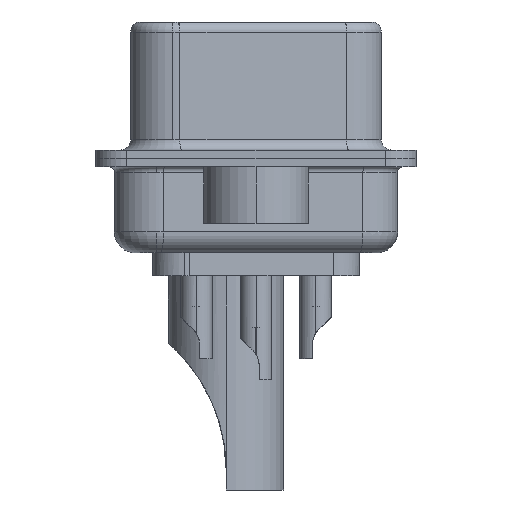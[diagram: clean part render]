
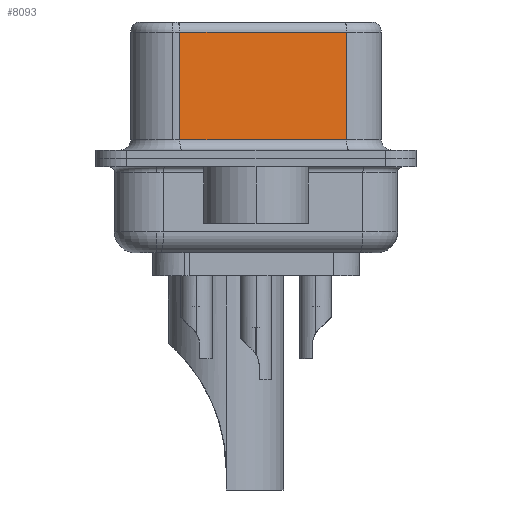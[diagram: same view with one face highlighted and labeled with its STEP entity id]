
A CAD part, left-side view. The second image highlights one B-rep face of the part: STEP entity #8093.
In plain terms, the highlighted planar face has unit normal (-0.985, -0.174, 0).
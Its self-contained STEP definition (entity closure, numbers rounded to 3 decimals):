
#473 = ORIENTED_EDGE ( 'NONE', *, *, #5941, .F. ) ;
#617 = LINE ( 'NONE', #20745, #11961 ) ;
#3370 = DIRECTION ( 'NONE',  ( -0.174, 0.985, 0. ) ) ;
#4381 = CARTESIAN_POINT ( 'NONE',  ( 3.73, 3.628, 6.02 ) ) ;
#4404 = AXIS2_PLACEMENT_3D ( 'NONE', #6633, #24317, #11160 ) ;
#4418 = PLANE ( 'NONE',  #4404 ) ;
#5811 = LINE ( 'NONE', #24162, #11006 ) ;
#5941 = EDGE_CURVE ( 'NONE', #20168, #17207, #21087, .T. ) ;
#6633 = CARTESIAN_POINT ( 'NONE',  ( 5.132, -4.322, 6.52 ) ) ;
#7620 = ORIENTED_EDGE ( 'NONE', *, *, #23532, .T. ) ;
#8022 = CARTESIAN_POINT ( 'NONE',  ( 5.132, -4.322, 6.02 ) ) ;
#8093 = ADVANCED_FACE ( 'NONE', ( #12339 ), #4418, .F. ) ;
#8444 = EDGE_CURVE ( 'NONE', #10817, #17207, #617, .T. ) ;
#9115 = VECTOR ( 'NONE', #3370, 1000. ) ;
#9285 = VERTEX_POINT ( 'NONE', #4381 ) ;
#10817 = VERTEX_POINT ( 'NONE', #13554 ) ;
#10947 = ORIENTED_EDGE ( 'NONE', *, *, #14185, .T. ) ;
#11006 = VECTOR ( 'NONE', #21976, 1000. ) ;
#11160 = DIRECTION ( 'NONE',  ( -0.174, 0.985, 0. ) ) ;
#11961 = VECTOR ( 'NONE', #27470, 1000. ) ;
#12339 = FACE_OUTER_BOUND ( 'NONE', #26367, .T. ) ;
#13116 = DIRECTION ( 'NONE',  ( 0., 0., -1. ) ) ;
#13554 = CARTESIAN_POINT ( 'NONE',  ( 3.73, 3.628, 0.9 ) ) ;
#13967 = CARTESIAN_POINT ( 'NONE',  ( 5.132, -4.322, 6.52 ) ) ;
#14185 = EDGE_CURVE ( 'NONE', #9285, #10817, #5811, .T. ) ;
#15232 = VECTOR ( 'NONE', #13116, 1000. ) ;
#17207 = VERTEX_POINT ( 'NONE', #24270 ) ;
#18881 = CARTESIAN_POINT ( 'NONE',  ( 5.132, -4.322, 6.02 ) ) ;
#20168 = VERTEX_POINT ( 'NONE', #8022 ) ;
#20745 = CARTESIAN_POINT ( 'NONE',  ( 5.132, -4.322, 0.9 ) ) ;
#21087 = LINE ( 'NONE', #13967, #15232 ) ;
#21459 = LINE ( 'NONE', #18881, #9115 ) ;
#21976 = DIRECTION ( 'NONE',  ( 0., 0., -1. ) ) ;
#23532 = EDGE_CURVE ( 'NONE', #20168, #9285, #21459, .T. ) ;
#24162 = CARTESIAN_POINT ( 'NONE',  ( 3.73, 3.628, 6.52 ) ) ;
#24270 = CARTESIAN_POINT ( 'NONE',  ( 5.132, -4.322, 0.9 ) ) ;
#24317 = DIRECTION ( 'NONE',  ( 0.985, 0.174, 0. ) ) ;
#25713 = ORIENTED_EDGE ( 'NONE', *, *, #8444, .T. ) ;
#26367 = EDGE_LOOP ( 'NONE', ( #473, #7620, #10947, #25713 ) ) ;
#27470 = DIRECTION ( 'NONE',  ( 0.174, -0.985, 0. ) ) ;
